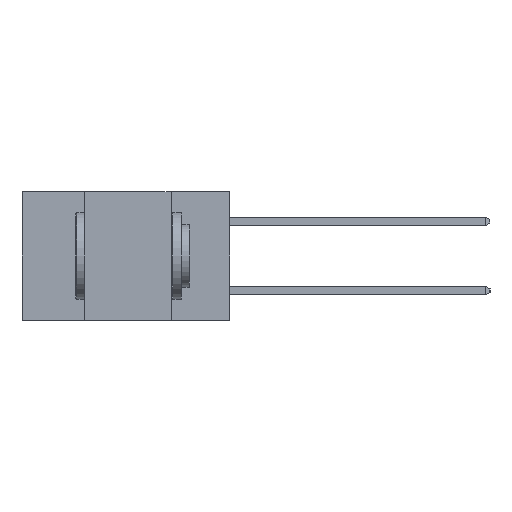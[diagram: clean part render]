
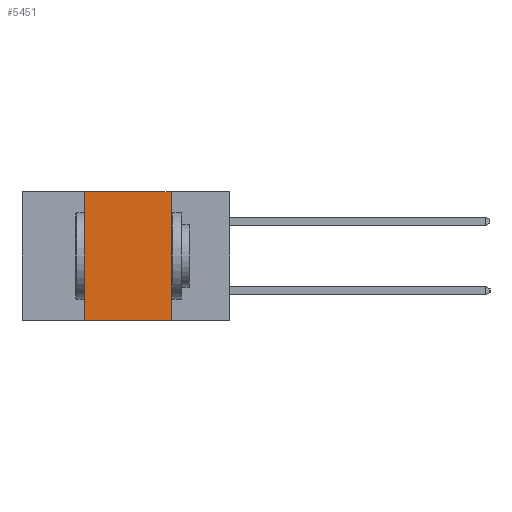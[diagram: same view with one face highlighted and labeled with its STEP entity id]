
A CAD part, left-side view. The second image highlights one B-rep face of the part: STEP entity #5451.
In plain terms, the highlighted planar face has unit normal (-1, 0, 0).
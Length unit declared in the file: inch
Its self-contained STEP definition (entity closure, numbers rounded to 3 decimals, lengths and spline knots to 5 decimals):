
#39 = VECTOR ( 'NONE', #7301, 39.37008 ) ;
#506 = EDGE_CURVE ( 'NONE', #9087, #9419, #11836, .T. ) ;
#542 = EDGE_CURVE ( 'NONE', #9087, #5298, #11304, .T. ) ;
#543 = EDGE_CURVE ( 'NONE', #5298, #4996, #4658, .T. ) ;
#552 = CARTESIAN_POINT ( 'NONE',  ( 0., 0.6, -0.37 ) ) ;
#607 = EDGE_CURVE ( 'NONE', #4996, #9419, #3480, .T. ) ;
#658 = FACE_OUTER_BOUND ( 'NONE', #3020, .T. ) ;
#732 = DIRECTION ( 'NONE',  ( 0., 0., -1. ) ) ;
#1694 = DIRECTION ( 'NONE',  ( 0., -1., 0. ) ) ;
#2239 = DIRECTION ( 'NONE',  ( 0., -1., 0. ) ) ;
#2469 = CARTESIAN_POINT ( 'NONE',  ( 0., 0.42, -0.37 ) ) ;
#2721 = AXIS2_PLACEMENT_3D ( 'NONE', #3772, #6548, #732 ) ;
#3020 = EDGE_LOOP ( 'NONE', ( #6204, #8245, #10997, #7556 ) ) ;
#3480 = LINE ( 'NONE', #4541, #39 ) ;
#3772 = CARTESIAN_POINT ( 'NONE',  ( 0., 0.6, 0. ) ) ;
#4094 = CARTESIAN_POINT ( 'NONE',  ( 0., 0.17, -0.37 ) ) ;
#4384 = VECTOR ( 'NONE', #8039, 39.37008 ) ;
#4541 = CARTESIAN_POINT ( 'NONE',  ( 0., 0.17, -0.37 ) ) ;
#4658 = LINE ( 'NONE', #9027, #11041 ) ;
#4996 = VERTEX_POINT ( 'NONE', #7579 ) ;
#5298 = VERTEX_POINT ( 'NONE', #11426 ) ;
#5451 = ADVANCED_FACE ( 'NONE', ( #658 ), #11644, .F. ) ;
#6204 = ORIENTED_EDGE ( 'NONE', *, *, #607, .F. ) ;
#6548 = DIRECTION ( 'NONE',  ( 1., 0., 0. ) ) ;
#7301 = DIRECTION ( 'NONE',  ( 0., 0., -1. ) ) ;
#7314 = CARTESIAN_POINT ( 'NONE',  ( 0., 0.42, -0.37 ) ) ;
#7349 = VECTOR ( 'NONE', #1694, 39.37008 ) ;
#7556 = ORIENTED_EDGE ( 'NONE', *, *, #506, .T. ) ;
#7579 = CARTESIAN_POINT ( 'NONE',  ( 0., 0.17, 0. ) ) ;
#8039 = DIRECTION ( 'NONE',  ( 0., 0., 1. ) ) ;
#8245 = ORIENTED_EDGE ( 'NONE', *, *, #543, .F. ) ;
#9027 = CARTESIAN_POINT ( 'NONE',  ( 0., 0.6, 0. ) ) ;
#9087 = VERTEX_POINT ( 'NONE', #7314 ) ;
#9419 = VERTEX_POINT ( 'NONE', #4094 ) ;
#10997 = ORIENTED_EDGE ( 'NONE', *, *, #542, .F. ) ;
#11041 = VECTOR ( 'NONE', #2239, 39.37008 ) ;
#11304 = LINE ( 'NONE', #2469, #4384 ) ;
#11426 = CARTESIAN_POINT ( 'NONE',  ( 0., 0.42, 0. ) ) ;
#11644 = PLANE ( 'NONE',  #2721 ) ;
#11836 = LINE ( 'NONE', #552, #7349 ) ;
